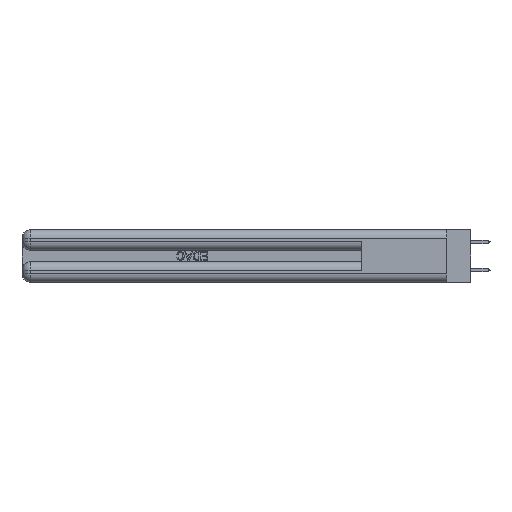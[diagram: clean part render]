
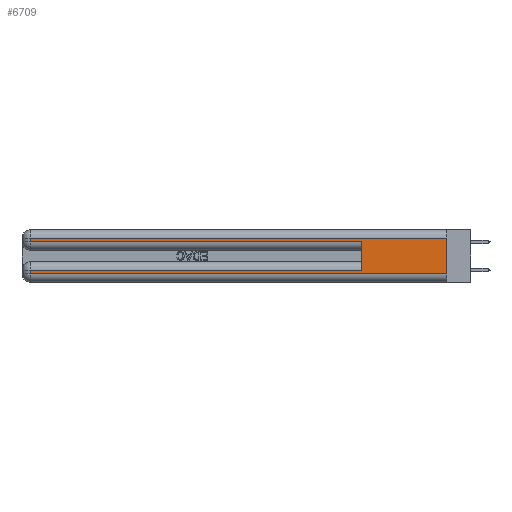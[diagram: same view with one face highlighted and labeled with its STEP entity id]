
A CAD part, left-side view. The second image highlights one B-rep face of the part: STEP entity #6709.
In plain terms, the highlighted planar face has unit normal (-1, 0, 0).
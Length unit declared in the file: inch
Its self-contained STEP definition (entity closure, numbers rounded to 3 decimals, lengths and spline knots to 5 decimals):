
#505 = LINE ( 'NONE', #12462, #33648 ) ;
#946 = LINE ( 'NONE', #5858, #11209 ) ;
#1000 = CARTESIAN_POINT ( 'NONE',  ( 0., 0., 0.37 ) ) ;
#1835 = LINE ( 'NONE', #14110, #9146 ) ;
#3027 = ORIENTED_EDGE ( 'NONE', *, *, #27808, .T. ) ;
#4144 = DIRECTION ( 'NONE',  ( 1., 0., 0. ) ) ;
#5275 = CARTESIAN_POINT ( 'NONE',  ( 0., 0., 0.085 ) ) ;
#5286 = VECTOR ( 'NONE', #36397, 39.37008 ) ;
#5349 = ORIENTED_EDGE ( 'NONE', *, *, #39284, .T. ) ;
#5761 = CARTESIAN_POINT ( 'NONE',  ( 0., 0., 0.37 ) ) ;
#5858 = CARTESIAN_POINT ( 'NONE',  ( 0., 0., 0.285 ) ) ;
#6543 = ORIENTED_EDGE ( 'NONE', *, *, #17958, .T. ) ;
#6709 = ADVANCED_FACE ( 'NONE', ( #8344 ), #19743, .F. ) ;
#7041 = VERTEX_POINT ( 'NONE', #12019 ) ;
#7298 = VERTEX_POINT ( 'NONE', #7376 ) ;
#7376 = CARTESIAN_POINT ( 'NONE',  ( 0., 2.94, 0.31 ) ) ;
#8344 = FACE_OUTER_BOUND ( 'NONE', #16097, .T. ) ;
#8607 = CARTESIAN_POINT ( 'NONE',  ( 0., 2.94, 0.06 ) ) ;
#8721 = VECTOR ( 'NONE', #36136, 39.37008 ) ;
#9081 = LINE ( 'NONE', #18302, #16487 ) ;
#9146 = VECTOR ( 'NONE', #38915, 39.37008 ) ;
#9336 = VERTEX_POINT ( 'NONE', #17863 ) ;
#9533 = ORIENTED_EDGE ( 'NONE', *, *, #17325, .F. ) ;
#9711 = LINE ( 'NONE', #11291, #8721 ) ;
#9823 = VERTEX_POINT ( 'NONE', #32765 ) ;
#11209 = VECTOR ( 'NONE', #12136, 39.37008 ) ;
#11243 = LINE ( 'NONE', #5761, #26917 ) ;
#11246 = DIRECTION ( 'NONE',  ( 0., -1., 0. ) ) ;
#11291 = CARTESIAN_POINT ( 'NONE',  ( 0., 0.6, 0.145 ) ) ;
#12019 = CARTESIAN_POINT ( 'NONE',  ( 0., 0., 0.06 ) ) ;
#12136 = DIRECTION ( 'NONE',  ( 0., -1., 0. ) ) ;
#12462 = CARTESIAN_POINT ( 'NONE',  ( 0., 0., 0.31 ) ) ;
#14110 = CARTESIAN_POINT ( 'NONE',  ( 0., 2.94, 0.37 ) ) ;
#14464 = AXIS2_PLACEMENT_3D ( 'NONE', #1000, #4144, #26033 ) ;
#14505 = EDGE_CURVE ( 'NONE', #31885, #7041, #22082, .T. ) ;
#15119 = ORIENTED_EDGE ( 'NONE', *, *, #37328, .T. ) ;
#16097 = EDGE_LOOP ( 'NONE', ( #19524, #15119, #6543, #34019, #9533, #5349, #3027, #18645 ) ) ;
#16487 = VECTOR ( 'NONE', #24611, 39.37008 ) ;
#16561 = EDGE_CURVE ( 'NONE', #9336, #7041, #11243, .T. ) ;
#17325 = EDGE_CURVE ( 'NONE', #9823, #38322, #9711, .T. ) ;
#17863 = CARTESIAN_POINT ( 'NONE',  ( 0., 0., 0.31 ) ) ;
#17958 = EDGE_CURVE ( 'NONE', #7298, #23636, #1835, .T. ) ;
#18302 = CARTESIAN_POINT ( 'NONE',  ( 0., 2.94, 0.37 ) ) ;
#18645 = ORIENTED_EDGE ( 'NONE', *, *, #14505, .T. ) ;
#19524 = ORIENTED_EDGE ( 'NONE', *, *, #16561, .F. ) ;
#19743 = PLANE ( 'NONE',  #14464 ) ;
#22082 = LINE ( 'NONE', #23863, #39421 ) ;
#22935 = LINE ( 'NONE', #5275, #5286 ) ;
#23465 = VERTEX_POINT ( 'NONE', #31234 ) ;
#23636 = VERTEX_POINT ( 'NONE', #35125 ) ;
#23863 = CARTESIAN_POINT ( 'NONE',  ( 0., 0., 0.06 ) ) ;
#24611 = DIRECTION ( 'NONE',  ( 0., 0., -1. ) ) ;
#26033 = DIRECTION ( 'NONE',  ( 0., 0., -1. ) ) ;
#26917 = VECTOR ( 'NONE', #33817, 39.37008 ) ;
#27808 = EDGE_CURVE ( 'NONE', #23465, #31885, #9081, .T. ) ;
#29124 = CARTESIAN_POINT ( 'NONE',  ( 0., 0.6, 0.285 ) ) ;
#31234 = CARTESIAN_POINT ( 'NONE',  ( 0., 2.94, 0.085 ) ) ;
#31885 = VERTEX_POINT ( 'NONE', #8607 ) ;
#32765 = CARTESIAN_POINT ( 'NONE',  ( 0., 0.6, 0.085 ) ) ;
#33648 = VECTOR ( 'NONE', #34221, 39.37008 ) ;
#33817 = DIRECTION ( 'NONE',  ( 0., 0., -1. ) ) ;
#34019 = ORIENTED_EDGE ( 'NONE', *, *, #38742, .T. ) ;
#34221 = DIRECTION ( 'NONE',  ( 0., 1., 0. ) ) ;
#35125 = CARTESIAN_POINT ( 'NONE',  ( 0., 2.94, 0.285 ) ) ;
#36136 = DIRECTION ( 'NONE',  ( 0., 0., 1. ) ) ;
#36397 = DIRECTION ( 'NONE',  ( 0., 1., 0. ) ) ;
#37328 = EDGE_CURVE ( 'NONE', #9336, #7298, #505, .T. ) ;
#38322 = VERTEX_POINT ( 'NONE', #29124 ) ;
#38742 = EDGE_CURVE ( 'NONE', #23636, #38322, #946, .T. ) ;
#38915 = DIRECTION ( 'NONE',  ( 0., 0., -1. ) ) ;
#39284 = EDGE_CURVE ( 'NONE', #9823, #23465, #22935, .T. ) ;
#39421 = VECTOR ( 'NONE', #11246, 39.37008 ) ;
